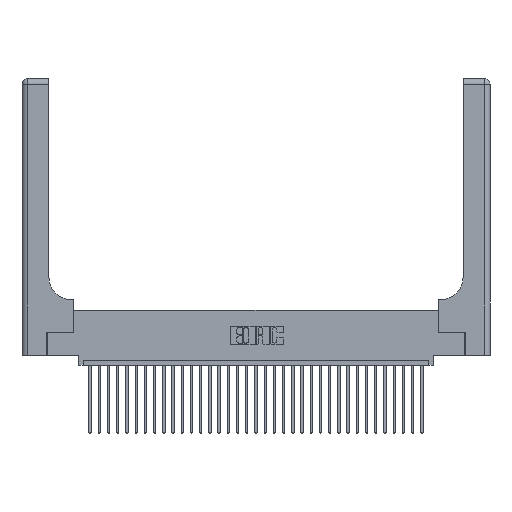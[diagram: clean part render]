
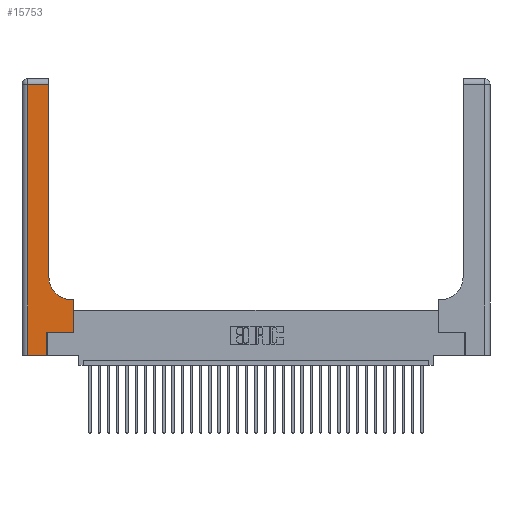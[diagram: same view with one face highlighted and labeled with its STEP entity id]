
A CAD part, top view. The second image highlights one B-rep face of the part: STEP entity #15753.
In plain terms, the highlighted planar face has unit normal (0, 0, 1).
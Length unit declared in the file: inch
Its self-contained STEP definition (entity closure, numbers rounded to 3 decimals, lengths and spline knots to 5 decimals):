
#933 = CARTESIAN_POINT ( 'NONE',  ( 0.06, 3., 0.37 ) ) ;
#1132 = CARTESIAN_POINT ( 'NONE',  ( 0.269, 0.25, 0.37 ) ) ;
#1457 = VECTOR ( 'NONE', #33224, 39.37008 ) ;
#1646 = LINE ( 'NONE', #933, #17481 ) ;
#2255 = VECTOR ( 'NONE', #5788, 39.37008 ) ;
#2452 = CIRCLE ( 'NONE', #33014, 0.25 ) ;
#2647 = EDGE_CURVE ( 'NONE', #8534, #26985, #10497, .T. ) ;
#3026 = CARTESIAN_POINT ( 'NONE',  ( 0.5415, 0.85, 0.37 ) ) ;
#4071 = DIRECTION ( 'NONE',  ( -1., 0., 0. ) ) ;
#4085 = VECTOR ( 'NONE', #17044, 39.37008 ) ;
#5788 = DIRECTION ( 'NONE',  ( 0., 1., 0. ) ) ;
#7095 = EDGE_CURVE ( 'NONE', #7238, #23981, #28018, .T. ) ;
#7161 = VECTOR ( 'NONE', #8245, 39.37008 ) ;
#7238 = VERTEX_POINT ( 'NONE', #30597 ) ;
#7520 = LINE ( 'NONE', #24908, #27159 ) ;
#8245 = DIRECTION ( 'NONE',  ( -1., 0., 0. ) ) ;
#8534 = VERTEX_POINT ( 'NONE', #11060 ) ;
#9545 = AXIS2_PLACEMENT_3D ( 'NONE', #11923, #17168, #4071 ) ;
#10067 = VERTEX_POINT ( 'NONE', #1132 ) ;
#10497 = LINE ( 'NONE', #21515, #17862 ) ;
#10966 = LINE ( 'NONE', #32783, #4085 ) ;
#11060 = CARTESIAN_POINT ( 'NONE',  ( 0.2915, 2.94, 0.37 ) ) ;
#11923 = CARTESIAN_POINT ( 'NONE',  ( 0., 3., 0.37 ) ) ;
#12111 = VERTEX_POINT ( 'NONE', #12958 ) ;
#12270 = CARTESIAN_POINT ( 'NONE',  ( 0.5585, 0.25, 0.37 ) ) ;
#12958 = CARTESIAN_POINT ( 'NONE',  ( 0.5585, 0.25, 0.37 ) ) ;
#13190 = EDGE_CURVE ( 'NONE', #23513, #10067, #29619, .T. ) ;
#13350 = EDGE_CURVE ( 'NONE', #27310, #23513, #7520, .T. ) ;
#13707 = ORIENTED_EDGE ( 'NONE', *, *, #23240, .T. ) ;
#13857 = FACE_OUTER_BOUND ( 'NONE', #24941, .T. ) ;
#13946 = ORIENTED_EDGE ( 'NONE', *, *, #7095, .T. ) ;
#14259 = ORIENTED_EDGE ( 'NONE', *, *, #13350, .T. ) ;
#15738 = DIRECTION ( 'NONE',  ( 1., 0., 0. ) ) ;
#15751 = EDGE_CURVE ( 'NONE', #18586, #8534, #10966, .T. ) ;
#15753 = ADVANCED_FACE ( 'NONE', ( #13857 ), #30024, .F. ) ;
#15956 = ORIENTED_EDGE ( 'NONE', *, *, #13190, .T. ) ;
#16537 = ORIENTED_EDGE ( 'NONE', *, *, #29536, .T. ) ;
#17044 = DIRECTION ( 'NONE',  ( 0., 1., 0. ) ) ;
#17072 = DIRECTION ( 'NONE',  ( 1., 0., 0. ) ) ;
#17168 = DIRECTION ( 'NONE',  ( 0., 0., -1. ) ) ;
#17481 = VECTOR ( 'NONE', #24668, 39.37008 ) ;
#17862 = VECTOR ( 'NONE', #21984, 39.37008 ) ;
#18021 = ORIENTED_EDGE ( 'NONE', *, *, #27023, .T. ) ;
#18586 = VERTEX_POINT ( 'NONE', #25437 ) ;
#21515 = CARTESIAN_POINT ( 'NONE',  ( 0., 2.94, 0.37 ) ) ;
#21666 = CARTESIAN_POINT ( 'NONE',  ( 0.269, 0., 0.37 ) ) ;
#21984 = DIRECTION ( 'NONE',  ( -1., 0., 0. ) ) ;
#23095 = LINE ( 'NONE', #12270, #1457 ) ;
#23240 = EDGE_CURVE ( 'NONE', #26985, #27310, #1646, .T. ) ;
#23513 = VERTEX_POINT ( 'NONE', #28178 ) ;
#23611 = DIRECTION ( 'NONE',  ( 1., 0., 0. ) ) ;
#23934 = CARTESIAN_POINT ( 'NONE',  ( 0.2915, 0.6, 0.37 ) ) ;
#23981 = VERTEX_POINT ( 'NONE', #25661 ) ;
#24668 = DIRECTION ( 'NONE',  ( 0., -1., 0. ) ) ;
#24908 = CARTESIAN_POINT ( 'NONE',  ( 0., 0., 0.37 ) ) ;
#24941 = EDGE_LOOP ( 'NONE', ( #31026, #33871, #13707, #14259, #15956, #32389, #18021, #13946, #16537 ) ) ;
#25437 = CARTESIAN_POINT ( 'NONE',  ( 0.2915, 0.85, 0.37 ) ) ;
#25661 = CARTESIAN_POINT ( 'NONE',  ( 0.5415, 0.6, 0.37 ) ) ;
#25974 = CARTESIAN_POINT ( 'NONE',  ( 0.269, 0.25, 0.37 ) ) ;
#26985 = VERTEX_POINT ( 'NONE', #30476 ) ;
#27023 = EDGE_CURVE ( 'NONE', #12111, #7238, #23095, .T. ) ;
#27159 = VECTOR ( 'NONE', #17072, 39.37008 ) ;
#27310 = VERTEX_POINT ( 'NONE', #29736 ) ;
#27339 = LINE ( 'NONE', #25974, #28166 ) ;
#28018 = LINE ( 'NONE', #23934, #7161 ) ;
#28166 = VECTOR ( 'NONE', #15738, 39.37008 ) ;
#28178 = CARTESIAN_POINT ( 'NONE',  ( 0.269, 0., 0.37 ) ) ;
#29536 = EDGE_CURVE ( 'NONE', #23981, #18586, #2452, .T. ) ;
#29619 = LINE ( 'NONE', #21666, #2255 ) ;
#29736 = CARTESIAN_POINT ( 'NONE',  ( 0.06, 0., 0.37 ) ) ;
#30024 = PLANE ( 'NONE',  #9545 ) ;
#30078 = EDGE_CURVE ( 'NONE', #10067, #12111, #27339, .T. ) ;
#30476 = CARTESIAN_POINT ( 'NONE',  ( 0.06, 2.94, 0.37 ) ) ;
#30597 = CARTESIAN_POINT ( 'NONE',  ( 0.5585, 0.6, 0.37 ) ) ;
#31026 = ORIENTED_EDGE ( 'NONE', *, *, #15751, .T. ) ;
#31398 = DIRECTION ( 'NONE',  ( 0., 0., -1. ) ) ;
#32389 = ORIENTED_EDGE ( 'NONE', *, *, #30078, .T. ) ;
#32783 = CARTESIAN_POINT ( 'NONE',  ( 0.2915, 3., 0.37 ) ) ;
#33014 = AXIS2_PLACEMENT_3D ( 'NONE', #3026, #31398, #23611 ) ;
#33224 = DIRECTION ( 'NONE',  ( 0., 1., 0. ) ) ;
#33871 = ORIENTED_EDGE ( 'NONE', *, *, #2647, .T. ) ;
